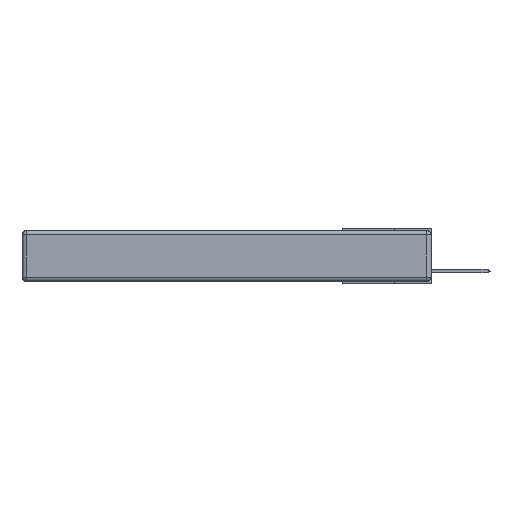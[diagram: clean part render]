
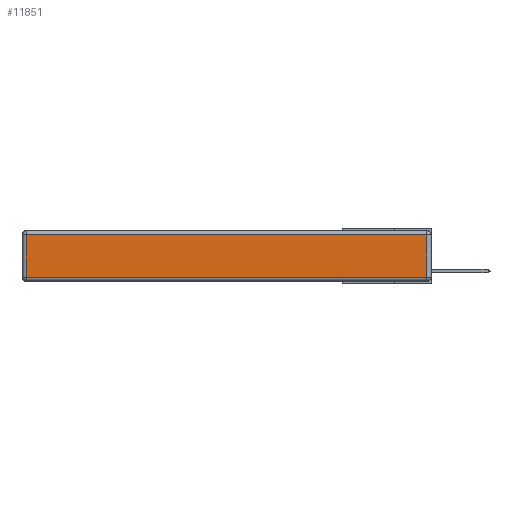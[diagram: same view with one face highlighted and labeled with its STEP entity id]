
A CAD part, left-side view. The second image highlights one B-rep face of the part: STEP entity #11851.
In plain terms, the highlighted planar face has unit normal (-1, 0, 0).
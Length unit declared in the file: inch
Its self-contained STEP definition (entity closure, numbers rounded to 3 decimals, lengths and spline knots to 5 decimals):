
#1576 = AXIS2_PLACEMENT_3D ( 'NONE', #25053, #25251, #11885 ) ;
#2679 = VECTOR ( 'NONE', #16567, 39.37008 ) ;
#4119 = CARTESIAN_POINT ( 'NONE',  ( 0., 2.72, -0.343 ) ) ;
#4860 = FACE_OUTER_BOUND ( 'NONE', #18713, .T. ) ;
#4900 = VERTEX_POINT ( 'NONE', #15157 ) ;
#5277 = DIRECTION ( 'NONE',  ( 0., -1., 0. ) ) ;
#6981 = VECTOR ( 'NONE', #25100, 39.37008 ) ;
#7759 = EDGE_CURVE ( 'NONE', #23648, #4900, #8590, .T. ) ;
#8508 = CARTESIAN_POINT ( 'NONE',  ( 0., 2.72, -0.313 ) ) ;
#8590 = LINE ( 'NONE', #14292, #2679 ) ;
#8810 = VECTOR ( 'NONE', #5277, 39.37008 ) ;
#9176 = CARTESIAN_POINT ( 'NONE',  ( 0., 0.03, -0.313 ) ) ;
#9428 = VERTEX_POINT ( 'NONE', #8508 ) ;
#9537 = PLANE ( 'NONE',  #1576 ) ;
#9793 = CARTESIAN_POINT ( 'NONE',  ( 0., 0.03, -0.03 ) ) ;
#11851 = ADVANCED_FACE ( 'NONE', ( #4860 ), #9537, .T. ) ;
#11885 = DIRECTION ( 'NONE',  ( 0., 0., 1. ) ) ;
#11987 = ORIENTED_EDGE ( 'NONE', *, *, #27597, .T. ) ;
#12271 = ORIENTED_EDGE ( 'NONE', *, *, #7759, .T. ) ;
#12969 = VECTOR ( 'NONE', #17450, 39.37008 ) ;
#14209 = ORIENTED_EDGE ( 'NONE', *, *, #23824, .T. ) ;
#14292 = CARTESIAN_POINT ( 'NONE',  ( 0., 2.75, -0.03 ) ) ;
#15157 = CARTESIAN_POINT ( 'NONE',  ( 0., 2.72, -0.03 ) ) ;
#16567 = DIRECTION ( 'NONE',  ( 0., 1., 0. ) ) ;
#16814 = EDGE_CURVE ( 'NONE', #17323, #23648, #27786, .T. ) ;
#17323 = VERTEX_POINT ( 'NONE', #9176 ) ;
#17450 = DIRECTION ( 'NONE',  ( 0., 0., -1. ) ) ;
#18713 = EDGE_LOOP ( 'NONE', ( #11987, #22108, #12271, #14209 ) ) ;
#22108 = ORIENTED_EDGE ( 'NONE', *, *, #16814, .T. ) ;
#22644 = CARTESIAN_POINT ( 'NONE',  ( 0., 0.03, -0.343 ) ) ;
#23648 = VERTEX_POINT ( 'NONE', #9793 ) ;
#23824 = EDGE_CURVE ( 'NONE', #4900, #9428, #24568, .T. ) ;
#24568 = LINE ( 'NONE', #4119, #12969 ) ;
#24982 = CARTESIAN_POINT ( 'NONE',  ( 0., 0., -0.313 ) ) ;
#25053 = CARTESIAN_POINT ( 'NONE',  ( 0., 0., -0.343 ) ) ;
#25100 = DIRECTION ( 'NONE',  ( 0., 0., 1. ) ) ;
#25251 = DIRECTION ( 'NONE',  ( -1., 0., 0. ) ) ;
#26786 = LINE ( 'NONE', #24982, #8810 ) ;
#27597 = EDGE_CURVE ( 'NONE', #9428, #17323, #26786, .T. ) ;
#27786 = LINE ( 'NONE', #22644, #6981 ) ;
